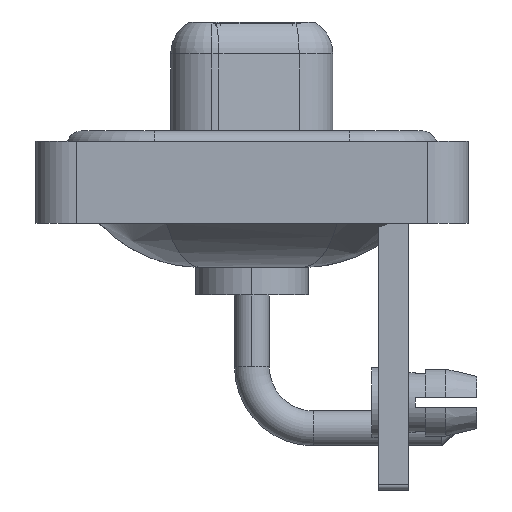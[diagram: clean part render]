
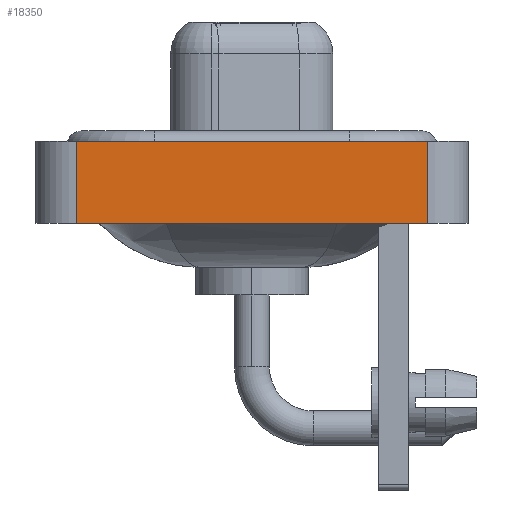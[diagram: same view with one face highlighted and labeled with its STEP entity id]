
A CAD part, left-side view. The second image highlights one B-rep face of the part: STEP entity #18350.
In plain terms, the highlighted planar face has unit normal (-1, 0, 0).
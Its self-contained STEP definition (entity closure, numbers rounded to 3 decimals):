
#29 = FACE_OUTER_BOUND ( 'NONE', #9342, .T. ) ;
#657 = CARTESIAN_POINT ( 'NONE',  ( -7.3, 8.55, -3.6 ) ) ;
#1428 = VECTOR ( 'NONE', #1835, 1000. ) ;
#1835 = DIRECTION ( 'NONE',  ( 0., -1., 0. ) ) ;
#2155 = LINE ( 'NONE', #16068, #5111 ) ;
#2822 = AXIS2_PLACEMENT_3D ( 'NONE', #7386, #19566, #13728 ) ;
#2987 = VERTEX_POINT ( 'NONE', #16833 ) ;
#4272 = CARTESIAN_POINT ( 'NONE',  ( -7.3, -8.55, 0.4 ) ) ;
#4370 = PLANE ( 'NONE',  #2822 ) ;
#4979 = CARTESIAN_POINT ( 'NONE',  ( -7.3, 8.55, -3.6 ) ) ;
#5111 = VECTOR ( 'NONE', #19273, 1000. ) ;
#5611 = DIRECTION ( 'NONE',  ( 0., 0., 1. ) ) ;
#6333 = CARTESIAN_POINT ( 'NONE',  ( -7.3, -8.55, -3.6 ) ) ;
#7386 = CARTESIAN_POINT ( 'NONE',  ( -7.3, -8.55, -3.6 ) ) ;
#7672 = VERTEX_POINT ( 'NONE', #6333 ) ;
#7990 = DIRECTION ( 'NONE',  ( 0., 0., 1. ) ) ;
#8078 = CARTESIAN_POINT ( 'NONE',  ( -7.3, -8.55, -3.6 ) ) ;
#9106 = ORIENTED_EDGE ( 'NONE', *, *, #18217, .F. ) ;
#9342 = EDGE_LOOP ( 'NONE', ( #19130, #9106, #11839, #16053 ) ) ;
#9474 = VECTOR ( 'NONE', #5611, 1000. ) ;
#10159 = LINE ( 'NONE', #11653, #9474 ) ;
#10614 = EDGE_CURVE ( 'NONE', #13076, #7672, #15652, .T. ) ;
#11653 = CARTESIAN_POINT ( 'NONE',  ( -7.3, -8.55, -3.6 ) ) ;
#11839 = ORIENTED_EDGE ( 'NONE', *, *, #12825, .F. ) ;
#11963 = VERTEX_POINT ( 'NONE', #4272 ) ;
#12344 = VECTOR ( 'NONE', #7990, 1000. ) ;
#12825 = EDGE_CURVE ( 'NONE', #13076, #2987, #18559, .T. ) ;
#13076 = VERTEX_POINT ( 'NONE', #657 ) ;
#13728 = DIRECTION ( 'NONE',  ( 0., 0., 1. ) ) ;
#15652 = LINE ( 'NONE', #8078, #1428 ) ;
#16053 = ORIENTED_EDGE ( 'NONE', *, *, #10614, .T. ) ;
#16068 = CARTESIAN_POINT ( 'NONE',  ( -7.3, -8.55, 0.4 ) ) ;
#16833 = CARTESIAN_POINT ( 'NONE',  ( -7.3, 8.55, 0.4 ) ) ;
#18217 = EDGE_CURVE ( 'NONE', #2987, #11963, #2155, .T. ) ;
#18350 = ADVANCED_FACE ( 'NONE', ( #29 ), #4370, .T. ) ;
#18559 = LINE ( 'NONE', #4979, #12344 ) ;
#19125 = EDGE_CURVE ( 'NONE', #7672, #11963, #10159, .T. ) ;
#19130 = ORIENTED_EDGE ( 'NONE', *, *, #19125, .T. ) ;
#19273 = DIRECTION ( 'NONE',  ( 0., -1., 0. ) ) ;
#19566 = DIRECTION ( 'NONE',  ( -1., 0., 0. ) ) ;
